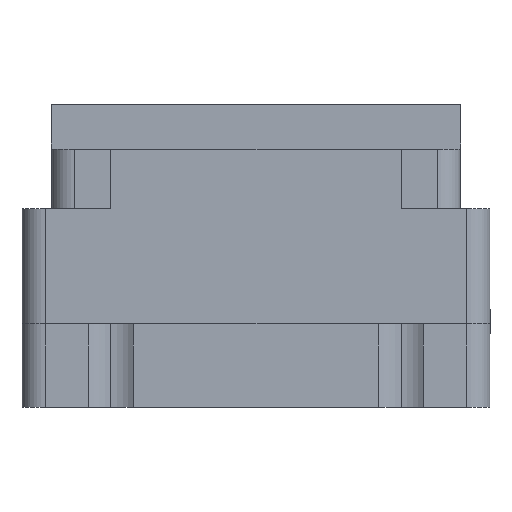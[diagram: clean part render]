
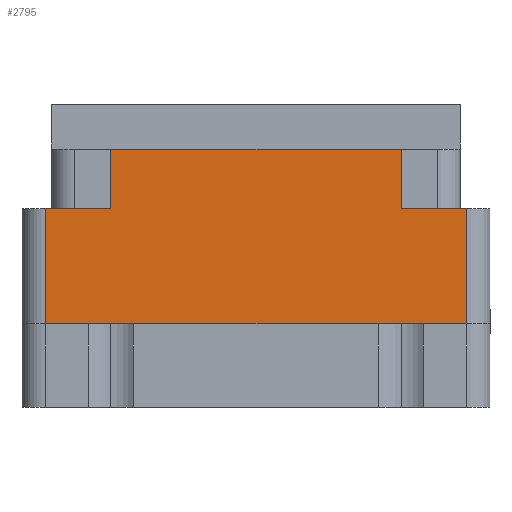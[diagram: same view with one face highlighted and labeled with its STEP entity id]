
A CAD part, left-side view. The second image highlights one B-rep face of the part: STEP entity #2795.
In plain terms, the highlighted planar face has unit normal (-1, 0, 0).
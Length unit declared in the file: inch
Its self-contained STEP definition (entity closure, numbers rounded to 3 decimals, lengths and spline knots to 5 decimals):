
#158 = CARTESIAN_POINT ( 'NONE',  ( -1.359, 0., -0.274 ) ) ;
#559 = LINE ( 'NONE', #56751, #53093 ) ;
#1621 = EDGE_CURVE ( 'NONE', #65125, #48977, #56651, .T. ) ;
#2528 = EDGE_LOOP ( 'NONE', ( #62138, #18846, #22084, #62784, #50136, #29298, #30240, #45990 ) ) ;
#2795 = ADVANCED_FACE ( 'NONE', ( #24781 ), #64751, .T. ) ;
#3619 = DIRECTION ( 'NONE',  ( 0., 0., 1. ) ) ;
#3831 = DIRECTION ( 'NONE',  ( -1., 0., 0. ) ) ;
#3872 = LINE ( 'NONE', #27069, #36426 ) ;
#5460 = LINE ( 'NONE', #64164, #44495 ) ;
#5799 = CARTESIAN_POINT ( 'NONE',  ( -1.359, -0.555, -0.798 ) ) ;
#6051 = CARTESIAN_POINT ( 'NONE',  ( -1.359, 0.555, -0.274 ) ) ;
#6876 = EDGE_CURVE ( 'NONE', #19255, #48977, #21093, .T. ) ;
#7015 = DIRECTION ( 'NONE',  ( 0., -1., 0. ) ) ;
#7857 = LINE ( 'NONE', #37959, #18256 ) ;
#10244 = EDGE_CURVE ( 'NONE', #34812, #65125, #5460, .T. ) ;
#15222 = CARTESIAN_POINT ( 'NONE',  ( -1.359, 0.555, -0.578 ) ) ;
#15685 = EDGE_CURVE ( 'NONE', #38743, #60131, #7857, .T. ) ;
#16199 = CARTESIAN_POINT ( 'NONE',  ( -1.359, 0.3825, -0.117 ) ) ;
#16602 = DIRECTION ( 'NONE',  ( 0., 0., 1. ) ) ;
#17248 = VERTEX_POINT ( 'NONE', #6051 ) ;
#17305 = CARTESIAN_POINT ( 'NONE',  ( -1.359, -0.3825, -0.274 ) ) ;
#17608 = VECTOR ( 'NONE', #37596, 39.37008 ) ;
#18256 = VECTOR ( 'NONE', #43557, 39.37008 ) ;
#18752 = CARTESIAN_POINT ( 'NONE',  ( -1.359, 0., -0.274 ) ) ;
#18846 = ORIENTED_EDGE ( 'NONE', *, *, #62537, .T. ) ;
#19255 = VERTEX_POINT ( 'NONE', #17305 ) ;
#21093 = LINE ( 'NONE', #18752, #44939 ) ;
#22084 = ORIENTED_EDGE ( 'NONE', *, *, #10244, .T. ) ;
#22086 = CARTESIAN_POINT ( 'NONE',  ( -1.359, 0.555, -0.798 ) ) ;
#23037 = VECTOR ( 'NONE', #45944, 39.37008 ) ;
#23578 = CARTESIAN_POINT ( 'NONE',  ( -1.359, -0.555, -0.274 ) ) ;
#24781 = FACE_OUTER_BOUND ( 'NONE', #2528, .T. ) ;
#27069 = CARTESIAN_POINT ( 'NONE',  ( -1.359, 0.617, -0.117 ) ) ;
#27101 = CARTESIAN_POINT ( 'NONE',  ( -1.359, -0.555, -0.578 ) ) ;
#27581 = EDGE_CURVE ( 'NONE', #60131, #31216, #3872, .T. ) ;
#29298 = ORIENTED_EDGE ( 'NONE', *, *, #36120, .T. ) ;
#30240 = ORIENTED_EDGE ( 'NONE', *, *, #27581, .F. ) ;
#31216 = VERTEX_POINT ( 'NONE', #39791 ) ;
#31531 = DIRECTION ( 'NONE',  ( 0., 0., 1. ) ) ;
#34812 = VERTEX_POINT ( 'NONE', #15222 ) ;
#35832 = LINE ( 'NONE', #22086, #17608 ) ;
#36120 = EDGE_CURVE ( 'NONE', #19255, #31216, #559, .T. ) ;
#36426 = VECTOR ( 'NONE', #7015, 39.37008 ) ;
#37596 = DIRECTION ( 'NONE',  ( 0., 0., -1. ) ) ;
#37959 = CARTESIAN_POINT ( 'NONE',  ( -1.359, 0.3825, -0.274 ) ) ;
#38743 = VERTEX_POINT ( 'NONE', #40124 ) ;
#39791 = CARTESIAN_POINT ( 'NONE',  ( -1.359, -0.3825, -0.117 ) ) ;
#40124 = CARTESIAN_POINT ( 'NONE',  ( -1.359, 0.3825, -0.274 ) ) ;
#43557 = DIRECTION ( 'NONE',  ( 0., 0., 1. ) ) ;
#44495 = VECTOR ( 'NONE', #49063, 39.37008 ) ;
#44939 = VECTOR ( 'NONE', #48935, 39.37008 ) ;
#45569 = EDGE_CURVE ( 'NONE', #17248, #38743, #50873, .T. ) ;
#45944 = DIRECTION ( 'NONE',  ( 0., -1., 0. ) ) ;
#45990 = ORIENTED_EDGE ( 'NONE', *, *, #15685, .F. ) ;
#48935 = DIRECTION ( 'NONE',  ( 0., -1., 0. ) ) ;
#48977 = VERTEX_POINT ( 'NONE', #23578 ) ;
#49063 = DIRECTION ( 'NONE',  ( 0., -1., 0. ) ) ;
#50136 = ORIENTED_EDGE ( 'NONE', *, *, #6876, .F. ) ;
#50873 = LINE ( 'NONE', #158, #23037 ) ;
#53093 = VECTOR ( 'NONE', #16602, 39.37008 ) ;
#54545 = CARTESIAN_POINT ( 'NONE',  ( -1.359, -0.617, -0.798 ) ) ;
#56651 = LINE ( 'NONE', #5799, #57422 ) ;
#56751 = CARTESIAN_POINT ( 'NONE',  ( -1.359, -0.3825, -0.274 ) ) ;
#57422 = VECTOR ( 'NONE', #31531, 39.37008 ) ;
#60131 = VERTEX_POINT ( 'NONE', #16199 ) ;
#62138 = ORIENTED_EDGE ( 'NONE', *, *, #45569, .F. ) ;
#62537 = EDGE_CURVE ( 'NONE', #17248, #34812, #35832, .T. ) ;
#62784 = ORIENTED_EDGE ( 'NONE', *, *, #1621, .T. ) ;
#63088 = AXIS2_PLACEMENT_3D ( 'NONE', #54545, #3831, #3619 ) ;
#64164 = CARTESIAN_POINT ( 'NONE',  ( -1.359, 0., -0.578 ) ) ;
#64751 = PLANE ( 'NONE',  #63088 ) ;
#65125 = VERTEX_POINT ( 'NONE', #27101 ) ;
